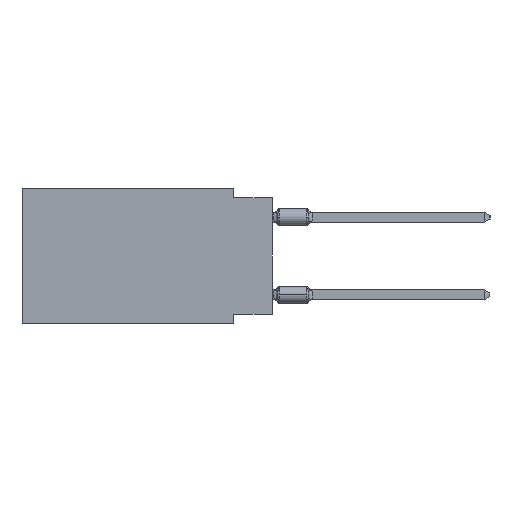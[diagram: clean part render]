
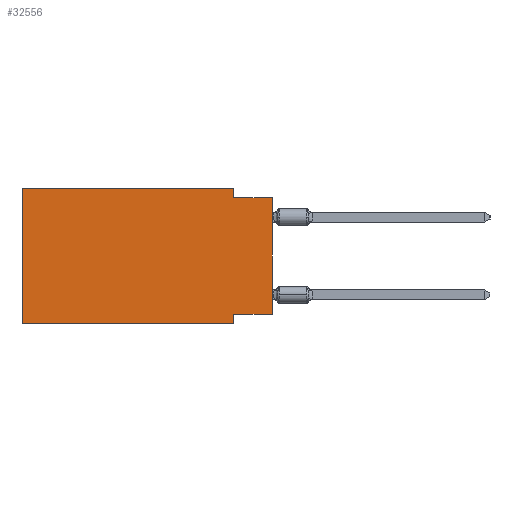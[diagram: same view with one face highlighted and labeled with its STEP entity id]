
A CAD part, left-side view. The second image highlights one B-rep face of the part: STEP entity #32556.
In plain terms, the highlighted planar face has unit normal (-1, 0, 0).
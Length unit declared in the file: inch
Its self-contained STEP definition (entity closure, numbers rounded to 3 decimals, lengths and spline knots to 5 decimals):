
#195 = VERTEX_POINT ( 'NONE', #11839 ) ;
#2148 = VECTOR ( 'NONE', #12126, 39.37008 ) ;
#2251 = ORIENTED_EDGE ( 'NONE', *, *, #11489, .F. ) ;
#3097 = CARTESIAN_POINT ( 'NONE',  ( 0., 0., -0.025 ) ) ;
#3687 = VERTEX_POINT ( 'NONE', #16735 ) ;
#4271 = ORIENTED_EDGE ( 'NONE', *, *, #7155, .T. ) ;
#4482 = VERTEX_POINT ( 'NONE', #13762 ) ;
#6082 = CARTESIAN_POINT ( 'NONE',  ( 0., 0.645, 0. ) ) ;
#7155 = EDGE_CURVE ( 'NONE', #3687, #7382, #27787, .T. ) ;
#7382 = VERTEX_POINT ( 'NONE', #36171 ) ;
#7640 = LINE ( 'NONE', #10666, #33043 ) ;
#7868 = CARTESIAN_POINT ( 'NONE',  ( 0., 0.645, 0. ) ) ;
#9746 = EDGE_CURVE ( 'NONE', #3687, #195, #37308, .T. ) ;
#10666 = CARTESIAN_POINT ( 'NONE',  ( 0., 0.1, 0. ) ) ;
#10798 = EDGE_CURVE ( 'NONE', #15205, #23041, #7640, .T. ) ;
#10899 = LINE ( 'NONE', #7868, #18040 ) ;
#11489 = EDGE_CURVE ( 'NONE', #195, #23619, #27048, .T. ) ;
#11839 = CARTESIAN_POINT ( 'NONE',  ( 0., 0.1, -0.325 ) ) ;
#12126 = DIRECTION ( 'NONE',  ( 0., 0., -1. ) ) ;
#13198 = DIRECTION ( 'NONE',  ( 0., 0., 1. ) ) ;
#13762 = CARTESIAN_POINT ( 'NONE',  ( 0., 0.645, 0. ) ) ;
#13832 = FACE_OUTER_BOUND ( 'NONE', #21263, .T. ) ;
#14958 = CARTESIAN_POINT ( 'NONE',  ( 0., 0.1, -0.35 ) ) ;
#15205 = VERTEX_POINT ( 'NONE', #34024 ) ;
#16081 = DIRECTION ( 'NONE',  ( 0., 0., 1. ) ) ;
#16172 = VECTOR ( 'NONE', #17116, 39.37008 ) ;
#16717 = VECTOR ( 'NONE', #36874, 39.37008 ) ;
#16735 = CARTESIAN_POINT ( 'NONE',  ( 0., 0., -0.325 ) ) ;
#17019 = VECTOR ( 'NONE', #34052, 39.37008 ) ;
#17116 = DIRECTION ( 'NONE',  ( 0., 1., 0. ) ) ;
#17176 = ORIENTED_EDGE ( 'NONE', *, *, #27383, .F. ) ;
#18028 = DIRECTION ( 'NONE',  ( 0., -1., 0. ) ) ;
#18040 = VECTOR ( 'NONE', #13198, 39.37008 ) ;
#19084 = EDGE_CURVE ( 'NONE', #4482, #15205, #23094, .T. ) ;
#19087 = VERTEX_POINT ( 'NONE', #19696 ) ;
#19334 = LINE ( 'NONE', #30870, #16717 ) ;
#19696 = CARTESIAN_POINT ( 'NONE',  ( 0., 0.645, -0.35 ) ) ;
#20328 = CARTESIAN_POINT ( 'NONE',  ( 0., 0., -0.325 ) ) ;
#20395 = VECTOR ( 'NONE', #18028, 39.37008 ) ;
#20938 = CARTESIAN_POINT ( 'NONE',  ( 0., 0.1, -0.35 ) ) ;
#21263 = EDGE_LOOP ( 'NONE', ( #4271, #17176, #26761, #21838, #34860, #30645, #2251, #31964 ) ) ;
#21763 = CARTESIAN_POINT ( 'NONE',  ( 0., 0., 0. ) ) ;
#21838 = ORIENTED_EDGE ( 'NONE', *, *, #19084, .F. ) ;
#22315 = PLANE ( 'NONE',  #27810 ) ;
#23041 = VERTEX_POINT ( 'NONE', #33646 ) ;
#23094 = LINE ( 'NONE', #6082, #17019 ) ;
#23619 = VERTEX_POINT ( 'NONE', #20938 ) ;
#25718 = DIRECTION ( 'NONE',  ( 0., 0., -1. ) ) ;
#26761 = ORIENTED_EDGE ( 'NONE', *, *, #10798, .F. ) ;
#27048 = LINE ( 'NONE', #14958, #2148 ) ;
#27383 = EDGE_CURVE ( 'NONE', #23041, #7382, #35205, .T. ) ;
#27787 = LINE ( 'NONE', #21763, #31069 ) ;
#27810 = AXIS2_PLACEMENT_3D ( 'NONE', #37006, #31182, #25718 ) ;
#30326 = DIRECTION ( 'NONE',  ( 0., 0., -1. ) ) ;
#30413 = EDGE_CURVE ( 'NONE', #19087, #4482, #10899, .T. ) ;
#30645 = ORIENTED_EDGE ( 'NONE', *, *, #36630, .T. ) ;
#30870 = CARTESIAN_POINT ( 'NONE',  ( 0., 0.645, -0.35 ) ) ;
#31069 = VECTOR ( 'NONE', #16081, 39.37008 ) ;
#31182 = DIRECTION ( 'NONE',  ( 1., 0., 0. ) ) ;
#31964 = ORIENTED_EDGE ( 'NONE', *, *, #9746, .F. ) ;
#32556 = ADVANCED_FACE ( 'NONE', ( #13832 ), #22315, .F. ) ;
#33043 = VECTOR ( 'NONE', #30326, 39.37008 ) ;
#33646 = CARTESIAN_POINT ( 'NONE',  ( 0., 0.1, -0.025 ) ) ;
#34024 = CARTESIAN_POINT ( 'NONE',  ( 0., 0.1, 0. ) ) ;
#34052 = DIRECTION ( 'NONE',  ( 0., -1., 0. ) ) ;
#34860 = ORIENTED_EDGE ( 'NONE', *, *, #30413, .F. ) ;
#35205 = LINE ( 'NONE', #3097, #20395 ) ;
#36171 = CARTESIAN_POINT ( 'NONE',  ( 0., 0., -0.025 ) ) ;
#36630 = EDGE_CURVE ( 'NONE', #19087, #23619, #19334, .T. ) ;
#36874 = DIRECTION ( 'NONE',  ( 0., -1., 0. ) ) ;
#37006 = CARTESIAN_POINT ( 'NONE',  ( 0., 0.645, 0. ) ) ;
#37308 = LINE ( 'NONE', #20328, #16172 ) ;
